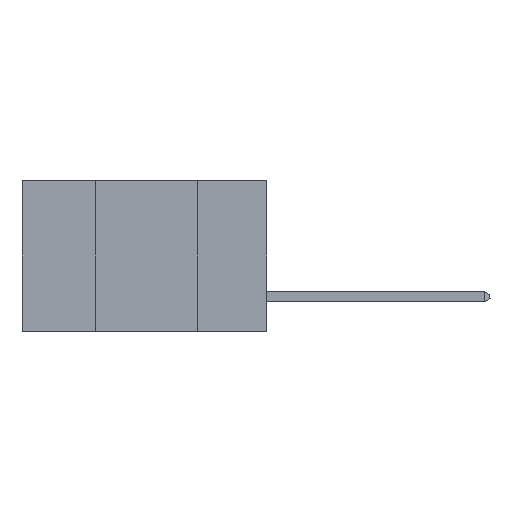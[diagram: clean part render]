
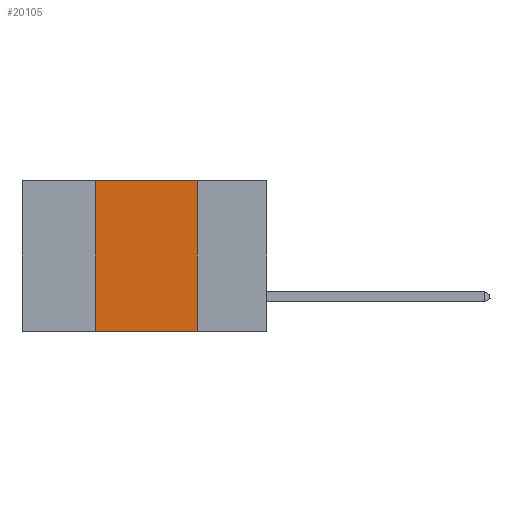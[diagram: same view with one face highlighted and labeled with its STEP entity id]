
A CAD part, left-side view. The second image highlights one B-rep face of the part: STEP entity #20105.
In plain terms, the highlighted planar face has unit normal (-1, 0, 0).
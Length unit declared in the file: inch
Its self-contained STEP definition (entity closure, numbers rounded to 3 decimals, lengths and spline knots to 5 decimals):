
#1914 = ORIENTED_EDGE ( 'NONE', *, *, #16367, .F. ) ;
#2019 = LINE ( 'NONE', #9459, #2622 ) ;
#2067 = ORIENTED_EDGE ( 'NONE', *, *, #6163, .T. ) ;
#2622 = VECTOR ( 'NONE', #9633, 39.37008 ) ;
#2770 = CARTESIAN_POINT ( 'NONE',  ( 0., 0.6, 0. ) ) ;
#3193 = EDGE_LOOP ( 'NONE', ( #9342, #1914, #10425, #2067 ) ) ;
#3930 = CARTESIAN_POINT ( 'NONE',  ( 0., 0.17, 0. ) ) ;
#4626 = VERTEX_POINT ( 'NONE', #20696 ) ;
#4751 = LINE ( 'NONE', #2770, #19287 ) ;
#6163 = EDGE_CURVE ( 'NONE', #4626, #17765, #24449, .T. ) ;
#7609 = VERTEX_POINT ( 'NONE', #20048 ) ;
#7884 = EDGE_CURVE ( 'NONE', #22054, #17765, #18725, .T. ) ;
#8148 = PLANE ( 'NONE',  #21890 ) ;
#8737 = DIRECTION ( 'NONE',  ( 0., -1., 0. ) ) ;
#9101 = DIRECTION ( 'NONE',  ( 0., -1., 0. ) ) ;
#9342 = ORIENTED_EDGE ( 'NONE', *, *, #7884, .F. ) ;
#9459 = CARTESIAN_POINT ( 'NONE',  ( 0., 0.42, 0. ) ) ;
#9633 = DIRECTION ( 'NONE',  ( 0., 0., 1. ) ) ;
#10101 = DIRECTION ( 'NONE',  ( 0., 0., -1. ) ) ;
#10425 = ORIENTED_EDGE ( 'NONE', *, *, #17457, .F. ) ;
#10816 = CARTESIAN_POINT ( 'NONE',  ( 0., 0.6, -0.37 ) ) ;
#11842 = FACE_OUTER_BOUND ( 'NONE', #3193, .T. ) ;
#11981 = CARTESIAN_POINT ( 'NONE',  ( 0., 0.6, 0. ) ) ;
#13606 = VECTOR ( 'NONE', #17078, 39.37008 ) ;
#14267 = CARTESIAN_POINT ( 'NONE',  ( 0., 0.17, -0.37 ) ) ;
#16367 = EDGE_CURVE ( 'NONE', #7609, #22054, #4751, .T. ) ;
#17078 = DIRECTION ( 'NONE',  ( 0., 0., -1. ) ) ;
#17457 = EDGE_CURVE ( 'NONE', #4626, #7609, #2019, .T. ) ;
#17765 = VERTEX_POINT ( 'NONE', #14267 ) ;
#18725 = LINE ( 'NONE', #3930, #13606 ) ;
#19287 = VECTOR ( 'NONE', #8737, 39.37008 ) ;
#19590 = DIRECTION ( 'NONE',  ( 1., 0., 0. ) ) ;
#20048 = CARTESIAN_POINT ( 'NONE',  ( 0., 0.42, 0. ) ) ;
#20105 = ADVANCED_FACE ( 'NONE', ( #11842 ), #8148, .F. ) ;
#20696 = CARTESIAN_POINT ( 'NONE',  ( 0., 0.42, -0.37 ) ) ;
#21890 = AXIS2_PLACEMENT_3D ( 'NONE', #11981, #19590, #10101 ) ;
#22054 = VERTEX_POINT ( 'NONE', #23499 ) ;
#23245 = VECTOR ( 'NONE', #9101, 39.37008 ) ;
#23499 = CARTESIAN_POINT ( 'NONE',  ( 0., 0.17, 0. ) ) ;
#24449 = LINE ( 'NONE', #10816, #23245 ) ;
